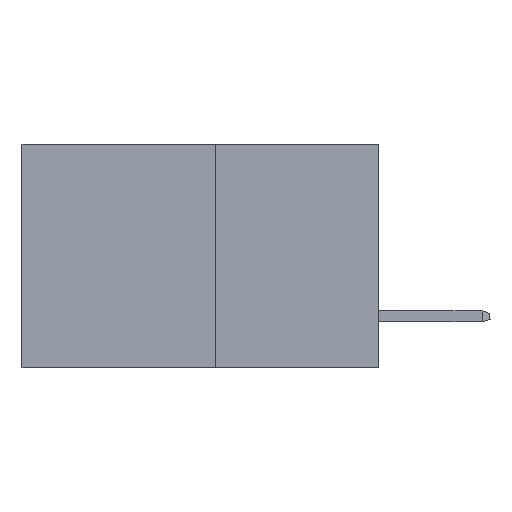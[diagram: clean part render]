
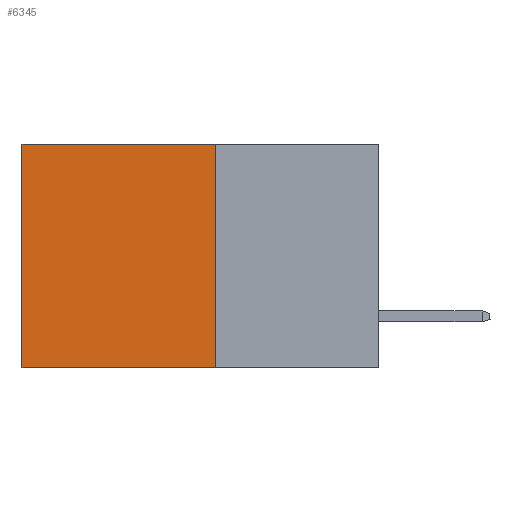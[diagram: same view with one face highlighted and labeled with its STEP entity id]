
A CAD part, left-side view. The second image highlights one B-rep face of the part: STEP entity #6345.
In plain terms, the highlighted planar face has unit normal (-1, 0, 0).
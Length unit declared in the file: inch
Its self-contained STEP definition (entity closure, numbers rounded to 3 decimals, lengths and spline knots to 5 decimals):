
#548 = CARTESIAN_POINT ( 'NONE',  ( 0.277, 0.27, -0.37 ) ) ;
#1432 = ORIENTED_EDGE ( 'NONE', *, *, #13652, .T. ) ;
#2481 = EDGE_CURVE ( 'NONE', #21699, #4649, #5827, .T. ) ;
#3643 = PLANE ( 'NONE',  #23476 ) ;
#4649 = VERTEX_POINT ( 'NONE', #5330 ) ;
#5185 = VECTOR ( 'NONE', #19588, 39.37008 ) ;
#5196 = VECTOR ( 'NONE', #12077, 39.37008 ) ;
#5330 = CARTESIAN_POINT ( 'NONE',  ( 0.277, 0.59, -0.37 ) ) ;
#5331 = CARTESIAN_POINT ( 'NONE',  ( 0.277, 0.27, 0. ) ) ;
#5812 = LINE ( 'NONE', #23040, #5185 ) ;
#5827 = LINE ( 'NONE', #21590, #5196 ) ;
#6345 = ADVANCED_FACE ( 'NONE', ( #7802 ), #3643, .F. ) ;
#7371 = DIRECTION ( 'NONE',  ( 0., 0., -1. ) ) ;
#7406 = CARTESIAN_POINT ( 'NONE',  ( 0.277, 0.27, -0.37 ) ) ;
#7802 = FACE_OUTER_BOUND ( 'NONE', #24386, .T. ) ;
#8375 = CARTESIAN_POINT ( 'NONE',  ( 0.277, 0.27, -0.37 ) ) ;
#8535 = VECTOR ( 'NONE', #20291, 39.37008 ) ;
#12076 = VERTEX_POINT ( 'NONE', #13287 ) ;
#12077 = DIRECTION ( 'NONE',  ( 0., 1., 0. ) ) ;
#13287 = CARTESIAN_POINT ( 'NONE',  ( 0.277, 0.59, 0. ) ) ;
#13652 = EDGE_CURVE ( 'NONE', #15467, #12076, #24001, .T. ) ;
#14827 = EDGE_CURVE ( 'NONE', #15467, #21699, #16702, .T. ) ;
#15467 = VERTEX_POINT ( 'NONE', #5331 ) ;
#15919 = ORIENTED_EDGE ( 'NONE', *, *, #20289, .T. ) ;
#16103 = VECTOR ( 'NONE', #7371, 39.37008 ) ;
#16702 = LINE ( 'NONE', #7406, #16103 ) ;
#18370 = ORIENTED_EDGE ( 'NONE', *, *, #2481, .F. ) ;
#19588 = DIRECTION ( 'NONE',  ( 0., 0., -1. ) ) ;
#20289 = EDGE_CURVE ( 'NONE', #12076, #4649, #5812, .T. ) ;
#20291 = DIRECTION ( 'NONE',  ( 0., 1., 0. ) ) ;
#20413 = CARTESIAN_POINT ( 'NONE',  ( 0.277, 0.27, 0. ) ) ;
#21590 = CARTESIAN_POINT ( 'NONE',  ( 0.277, 0.27, -0.37 ) ) ;
#21699 = VERTEX_POINT ( 'NONE', #8375 ) ;
#23040 = CARTESIAN_POINT ( 'NONE',  ( 0.277, 0.59, -0.37 ) ) ;
#23476 = AXIS2_PLACEMENT_3D ( 'NONE', #548, #25250, #25242 ) ;
#24001 = LINE ( 'NONE', #20413, #8535 ) ;
#24386 = EDGE_LOOP ( 'NONE', ( #15919, #18370, #24532, #1432 ) ) ;
#24532 = ORIENTED_EDGE ( 'NONE', *, *, #14827, .F. ) ;
#25242 = DIRECTION ( 'NONE',  ( 0., 0., -1. ) ) ;
#25250 = DIRECTION ( 'NONE',  ( 1., 0., 0. ) ) ;
